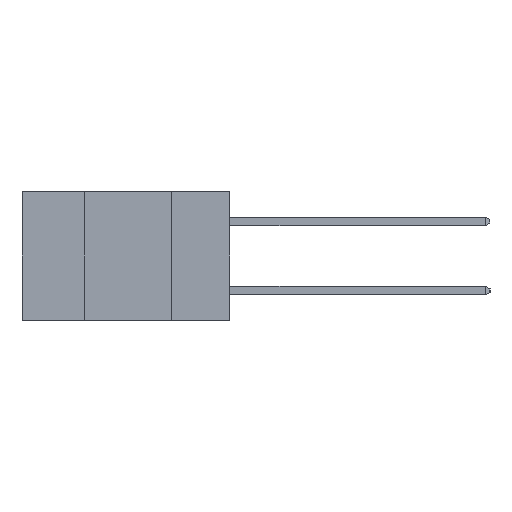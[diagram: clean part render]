
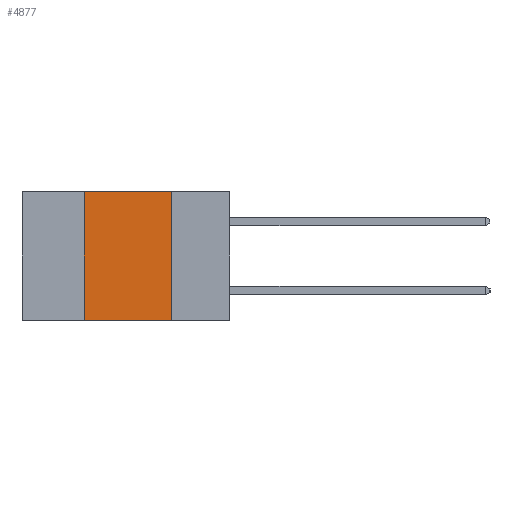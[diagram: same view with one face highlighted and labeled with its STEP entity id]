
A CAD part, left-side view. The second image highlights one B-rep face of the part: STEP entity #4877.
In plain terms, the highlighted planar face has unit normal (-1, 0, 0).
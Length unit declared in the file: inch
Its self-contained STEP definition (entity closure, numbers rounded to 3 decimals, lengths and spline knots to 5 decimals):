
#333 = ORIENTED_EDGE ( 'NONE', *, *, #7519, .F. ) ;
#722 = EDGE_LOOP ( 'NONE', ( #16013, #333, #17461, #1127 ) ) ;
#867 = DIRECTION ( 'NONE',  ( 0., 0., 1. ) ) ;
#1127 = ORIENTED_EDGE ( 'NONE', *, *, #6840, .T. ) ;
#1185 = CARTESIAN_POINT ( 'NONE',  ( 0., 0.42, -0.37 ) ) ;
#1220 = CARTESIAN_POINT ( 'NONE',  ( 0., 0.17, -0.37 ) ) ;
#2660 = LINE ( 'NONE', #1185, #19678 ) ;
#2907 = DIRECTION ( 'NONE',  ( 0., -1., 0. ) ) ;
#4551 = VERTEX_POINT ( 'NONE', #11212 ) ;
#4877 = ADVANCED_FACE ( 'NONE', ( #18708 ), #6301, .F. ) ;
#5294 = CARTESIAN_POINT ( 'NONE',  ( 0., 0.42, 0. ) ) ;
#5324 = EDGE_CURVE ( 'NONE', #20801, #6488, #2660, .T. ) ;
#6269 = DIRECTION ( 'NONE',  ( 0., 0., -1. ) ) ;
#6296 = DIRECTION ( 'NONE',  ( 1., 0., 0. ) ) ;
#6301 = PLANE ( 'NONE',  #18316 ) ;
#6370 = CARTESIAN_POINT ( 'NONE',  ( 0., 0.6, 0. ) ) ;
#6488 = VERTEX_POINT ( 'NONE', #5294 ) ;
#6840 = EDGE_CURVE ( 'NONE', #20801, #4551, #16128, .T. ) ;
#7346 = VECTOR ( 'NONE', #16164, 39.37008 ) ;
#7519 = EDGE_CURVE ( 'NONE', #6488, #14600, #15839, .T. ) ;
#7915 = CARTESIAN_POINT ( 'NONE',  ( 0., 0.6, 0. ) ) ;
#9882 = LINE ( 'NONE', #1220, #21222 ) ;
#10917 = EDGE_CURVE ( 'NONE', #14600, #4551, #9882, .T. ) ;
#11181 = DIRECTION ( 'NONE',  ( 0., 0., -1. ) ) ;
#11212 = CARTESIAN_POINT ( 'NONE',  ( 0., 0.17, -0.37 ) ) ;
#12310 = CARTESIAN_POINT ( 'NONE',  ( 0., 0.42, -0.37 ) ) ;
#14600 = VERTEX_POINT ( 'NONE', #14744 ) ;
#14744 = CARTESIAN_POINT ( 'NONE',  ( 0., 0.17, 0. ) ) ;
#15839 = LINE ( 'NONE', #7915, #19582 ) ;
#16013 = ORIENTED_EDGE ( 'NONE', *, *, #10917, .F. ) ;
#16128 = LINE ( 'NONE', #20884, #7346 ) ;
#16164 = DIRECTION ( 'NONE',  ( 0., -1., 0. ) ) ;
#17461 = ORIENTED_EDGE ( 'NONE', *, *, #5324, .F. ) ;
#18316 = AXIS2_PLACEMENT_3D ( 'NONE', #6370, #6296, #6269 ) ;
#18708 = FACE_OUTER_BOUND ( 'NONE', #722, .T. ) ;
#19582 = VECTOR ( 'NONE', #2907, 39.37008 ) ;
#19678 = VECTOR ( 'NONE', #867, 39.37008 ) ;
#20801 = VERTEX_POINT ( 'NONE', #12310 ) ;
#20884 = CARTESIAN_POINT ( 'NONE',  ( 0., 0.6, -0.37 ) ) ;
#21222 = VECTOR ( 'NONE', #11181, 39.37008 ) ;
